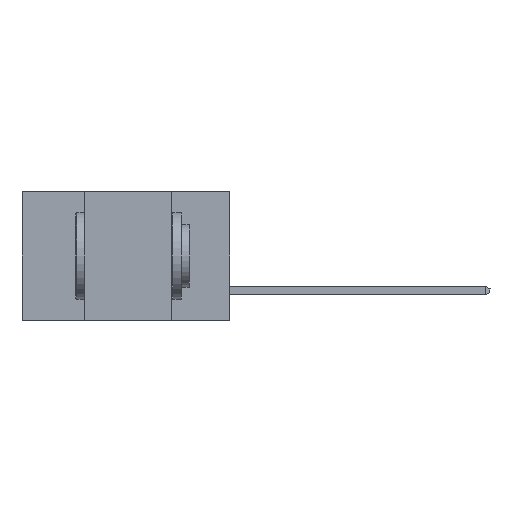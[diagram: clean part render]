
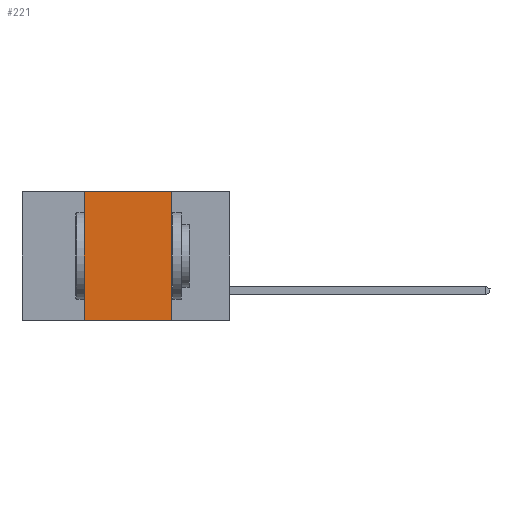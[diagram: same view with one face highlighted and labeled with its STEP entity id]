
A CAD part, left-side view. The second image highlights one B-rep face of the part: STEP entity #221.
In plain terms, the highlighted planar face has unit normal (-1, 0, 0).
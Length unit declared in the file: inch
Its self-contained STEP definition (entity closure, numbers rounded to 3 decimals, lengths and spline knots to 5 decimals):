
#221 = ADVANCED_FACE ( 'NONE', ( #8638 ), #24568, .F. ) ;
#1142 = DIRECTION ( 'NONE',  ( 0., 0., -1. ) ) ;
#1240 = VECTOR ( 'NONE', #14092, 39.37008 ) ;
#2142 = DIRECTION ( 'NONE',  ( 0., -1., 0. ) ) ;
#2493 = AXIS2_PLACEMENT_3D ( 'NONE', #20375, #6542, #10351 ) ;
#3000 = ORIENTED_EDGE ( 'NONE', *, *, #18191, .F. ) ;
#3662 = VERTEX_POINT ( 'NONE', #10951 ) ;
#4911 = EDGE_CURVE ( 'NONE', #3662, #6044, #15497, .T. ) ;
#4984 = CARTESIAN_POINT ( 'NONE',  ( 0., 0.42, 0. ) ) ;
#6044 = VERTEX_POINT ( 'NONE', #13966 ) ;
#6542 = DIRECTION ( 'NONE',  ( 1., 0., 0. ) ) ;
#6620 = CARTESIAN_POINT ( 'NONE',  ( 0., 0.6, -0.37 ) ) ;
#6957 = VERTEX_POINT ( 'NONE', #12313 ) ;
#8638 = FACE_OUTER_BOUND ( 'NONE', #15146, .T. ) ;
#10351 = DIRECTION ( 'NONE',  ( 0., 0., -1. ) ) ;
#10490 = VECTOR ( 'NONE', #23521, 39.37008 ) ;
#10951 = CARTESIAN_POINT ( 'NONE',  ( 0., 0.17, 0. ) ) ;
#11408 = LINE ( 'NONE', #15495, #10490 ) ;
#12006 = VECTOR ( 'NONE', #1142, 39.37008 ) ;
#12134 = EDGE_CURVE ( 'NONE', #6957, #6044, #18349, .T. ) ;
#12232 = ORIENTED_EDGE ( 'NONE', *, *, #12134, .T. ) ;
#12313 = CARTESIAN_POINT ( 'NONE',  ( 0., 0.42, -0.37 ) ) ;
#13966 = CARTESIAN_POINT ( 'NONE',  ( 0., 0.17, -0.37 ) ) ;
#14092 = DIRECTION ( 'NONE',  ( 0., 0., 1. ) ) ;
#15146 = EDGE_LOOP ( 'NONE', ( #24784, #19497, #3000, #12232 ) ) ;
#15495 = CARTESIAN_POINT ( 'NONE',  ( 0., 0.6, 0. ) ) ;
#15497 = LINE ( 'NONE', #23134, #12006 ) ;
#17799 = EDGE_CURVE ( 'NONE', #20860, #3662, #11408, .T. ) ;
#18191 = EDGE_CURVE ( 'NONE', #6957, #20860, #20300, .T. ) ;
#18349 = LINE ( 'NONE', #6620, #18375 ) ;
#18375 = VECTOR ( 'NONE', #2142, 39.37008 ) ;
#19497 = ORIENTED_EDGE ( 'NONE', *, *, #17799, .F. ) ;
#20300 = LINE ( 'NONE', #25676, #1240 ) ;
#20375 = CARTESIAN_POINT ( 'NONE',  ( 0., 0.6, 0. ) ) ;
#20860 = VERTEX_POINT ( 'NONE', #4984 ) ;
#23134 = CARTESIAN_POINT ( 'NONE',  ( 0., 0.17, -0.37 ) ) ;
#23521 = DIRECTION ( 'NONE',  ( 0., -1., 0. ) ) ;
#24568 = PLANE ( 'NONE',  #2493 ) ;
#24784 = ORIENTED_EDGE ( 'NONE', *, *, #4911, .F. ) ;
#25676 = CARTESIAN_POINT ( 'NONE',  ( 0., 0.42, -0.37 ) ) ;
